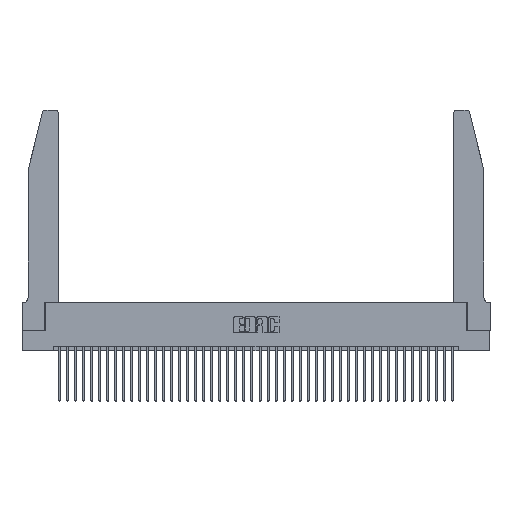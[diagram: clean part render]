
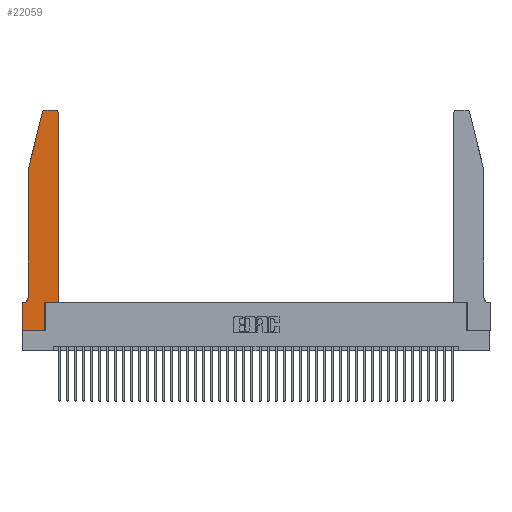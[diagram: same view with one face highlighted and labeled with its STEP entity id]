
A CAD part, top view. The second image highlights one B-rep face of the part: STEP entity #22059.
In plain terms, the highlighted planar face has unit normal (0, 0, 1).
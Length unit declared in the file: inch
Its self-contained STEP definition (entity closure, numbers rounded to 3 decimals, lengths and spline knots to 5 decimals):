
#1472 = CARTESIAN_POINT ( 'NONE',  ( 0.4505, 0.35, 0.37 ) ) ;
#2351 = ORIENTED_EDGE ( 'NONE', *, *, #39076, .T. ) ;
#2906 = DIRECTION ( 'NONE',  ( 0., -1., 0. ) ) ;
#3078 = LINE ( 'NONE', #39108, #34207 ) ;
#3206 = DIRECTION ( 'NONE',  ( 0., 0., 1. ) ) ;
#3647 = CARTESIAN_POINT ( 'NONE',  ( 0.4505, 2.72, 0.37 ) ) ;
#4287 = EDGE_CURVE ( 'NONE', #18039, #28074, #35984, .T. ) ;
#4755 = VERTEX_POINT ( 'NONE', #15818 ) ;
#5447 = LINE ( 'NONE', #38028, #14300 ) ;
#5801 = DIRECTION ( 'NONE',  ( 1., 0., 0. ) ) ;
#5887 = CARTESIAN_POINT ( 'NONE',  ( 0., 0., 0.37 ) ) ;
#7144 = CARTESIAN_POINT ( 'NONE',  ( 0.0055, 0.42, 0.37 ) ) ;
#7208 = EDGE_CURVE ( 'NONE', #29296, #27183, #28351, .T. ) ;
#7875 = DIRECTION ( 'NONE',  ( 0., 0., -1. ) ) ;
#8440 = VERTEX_POINT ( 'NONE', #33783 ) ;
#8445 = VECTOR ( 'NONE', #2906, 39.37008 ) ;
#8451 = ORIENTED_EDGE ( 'NONE', *, *, #24967, .T. ) ;
#8682 = DIRECTION ( 'NONE',  ( -1., 0., 0. ) ) ;
#8782 = CIRCLE ( 'NONE', #34345, 0.03 ) ;
#8792 = ORIENTED_EDGE ( 'NONE', *, *, #20204, .T. ) ;
#8974 = CARTESIAN_POINT ( 'NONE',  ( 0.2605, 2.75, 0.37 ) ) ;
#9156 = PLANE ( 'NONE',  #19993 ) ;
#9279 = DIRECTION ( 'NONE',  ( 0., 1., 0. ) ) ;
#9393 = VECTOR ( 'NONE', #8682, 39.37008 ) ;
#9702 = DIRECTION ( 'NONE',  ( 1., 0., 0. ) ) ;
#9722 = CARTESIAN_POINT ( 'NONE',  ( 0.4505, 0.35, 0.37 ) ) ;
#10453 = CARTESIAN_POINT ( 'NONE',  ( 0.2865, 0., 0.37 ) ) ;
#10726 = VERTEX_POINT ( 'NONE', #31061 ) ;
#10952 = VERTEX_POINT ( 'NONE', #1472 ) ;
#12100 = EDGE_LOOP ( 'NONE', ( #17981, #35621, #13462, #32931, #8792, #8451, #27539, #33921, #13154, #21253, #2351, #29216 ) ) ;
#12704 = EDGE_CURVE ( 'NONE', #29987, #22863, #8782, .T. ) ;
#13154 = ORIENTED_EDGE ( 'NONE', *, *, #7208, .T. ) ;
#13342 = VECTOR ( 'NONE', #42743, 39.37008 ) ;
#13364 = EDGE_CURVE ( 'NONE', #27407, #18039, #17043, .T. ) ;
#13462 = ORIENTED_EDGE ( 'NONE', *, *, #13364, .T. ) ;
#14059 = DIRECTION ( 'NONE',  ( -1., 0., 0. ) ) ;
#14300 = VECTOR ( 'NONE', #21576, 39.37008 ) ;
#14348 = CARTESIAN_POINT ( 'NONE',  ( 0., 0.35, 0.37 ) ) ;
#14452 = VECTOR ( 'NONE', #19868, 39.37008 ) ;
#14802 = EDGE_CURVE ( 'NONE', #19321, #10726, #39784, .T. ) ;
#15228 = EDGE_CURVE ( 'NONE', #22863, #8440, #37889, .T. ) ;
#15280 = CARTESIAN_POINT ( 'NONE',  ( 0.4205, 2.72, 0.37 ) ) ;
#15305 = VECTOR ( 'NONE', #40096, 39.37008 ) ;
#15593 = LINE ( 'NONE', #9722, #17670 ) ;
#15818 = CARTESIAN_POINT ( 'NONE',  ( 0.0055, 0.35, 0.37 ) ) ;
#16521 = EDGE_CURVE ( 'NONE', #27183, #10952, #3078, .T. ) ;
#17043 = LINE ( 'NONE', #29581, #14452 ) ;
#17247 = CARTESIAN_POINT ( 'NONE',  ( 0.0755, 0.35, 0.37 ) ) ;
#17670 = VECTOR ( 'NONE', #9279, 39.37008 ) ;
#17981 = ORIENTED_EDGE ( 'NONE', *, *, #15228, .T. ) ;
#18039 = VERTEX_POINT ( 'NONE', #24768 ) ;
#18991 = VECTOR ( 'NONE', #14059, 39.37008 ) ;
#19063 = AXIS2_PLACEMENT_3D ( 'NONE', #7144, #7875, #31136 ) ;
#19321 = VERTEX_POINT ( 'NONE', #14348 ) ;
#19694 = DIRECTION ( 'NONE',  ( 0., 0., 1. ) ) ;
#19805 = CARTESIAN_POINT ( 'NONE',  ( 0., 0.35, 0.37 ) ) ;
#19868 = DIRECTION ( 'NONE',  ( -0.239, -0.971, 0. ) ) ;
#19993 = AXIS2_PLACEMENT_3D ( 'NONE', #19805, #3206, #5801 ) ;
#20038 = CARTESIAN_POINT ( 'NONE',  ( 0.284, 2.72, 0.37 ) ) ;
#20204 = EDGE_CURVE ( 'NONE', #28074, #4755, #42888, .T. ) ;
#21104 = LINE ( 'NONE', #17247, #18991 ) ;
#21253 = ORIENTED_EDGE ( 'NONE', *, *, #16521, .T. ) ;
#21576 = DIRECTION ( 'NONE',  ( 1., 0., 0. ) ) ;
#22059 = ADVANCED_FACE ( 'NONE', ( #37833 ), #9156, .T. ) ;
#22174 = CIRCLE ( 'NONE', #38013, 0.03 ) ;
#22736 = DIRECTION ( 'NONE',  ( 1., 0., 0. ) ) ;
#22843 = CARTESIAN_POINT ( 'NONE',  ( 0.0755, 0.42, 0.37 ) ) ;
#22863 = VERTEX_POINT ( 'NONE', #23875 ) ;
#23875 = CARTESIAN_POINT ( 'NONE',  ( 0.4205, 2.75, 0.37 ) ) ;
#23933 = CARTESIAN_POINT ( 'NONE',  ( 0.0755, 2., 0.37 ) ) ;
#24768 = CARTESIAN_POINT ( 'NONE',  ( 0.0755, 2., 0.37 ) ) ;
#24967 = EDGE_CURVE ( 'NONE', #4755, #19321, #21104, .T. ) ;
#27183 = VERTEX_POINT ( 'NONE', #36464 ) ;
#27407 = VERTEX_POINT ( 'NONE', #31963 ) ;
#27539 = ORIENTED_EDGE ( 'NONE', *, *, #14802, .T. ) ;
#28074 = VERTEX_POINT ( 'NONE', #22843 ) ;
#28351 = LINE ( 'NONE', #30420, #15305 ) ;
#29216 = ORIENTED_EDGE ( 'NONE', *, *, #12704, .T. ) ;
#29296 = VERTEX_POINT ( 'NONE', #10453 ) ;
#29581 = CARTESIAN_POINT ( 'NONE',  ( 0.0755, 2., 0.37 ) ) ;
#29895 = DIRECTION ( 'NONE',  ( 0., 0., 1. ) ) ;
#29987 = VERTEX_POINT ( 'NONE', #3647 ) ;
#30420 = CARTESIAN_POINT ( 'NONE',  ( 0.2865, 0.35, 0.37 ) ) ;
#31061 = CARTESIAN_POINT ( 'NONE',  ( 0., 0., 0.37 ) ) ;
#31136 = DIRECTION ( 'NONE',  ( -1., 0., 0. ) ) ;
#31963 = CARTESIAN_POINT ( 'NONE',  ( 0.25487, 2.72718, 0.37 ) ) ;
#32931 = ORIENTED_EDGE ( 'NONE', *, *, #4287, .T. ) ;
#33783 = CARTESIAN_POINT ( 'NONE',  ( 0.284, 2.75, 0.37 ) ) ;
#33921 = ORIENTED_EDGE ( 'NONE', *, *, #42548, .T. ) ;
#34207 = VECTOR ( 'NONE', #9702, 39.37008 ) ;
#34345 = AXIS2_PLACEMENT_3D ( 'NONE', #15280, #19694, #22736 ) ;
#35621 = ORIENTED_EDGE ( 'NONE', *, *, #35917, .T. ) ;
#35917 = EDGE_CURVE ( 'NONE', #8440, #27407, #22174, .T. ) ;
#35984 = LINE ( 'NONE', #23933, #8445 ) ;
#36464 = CARTESIAN_POINT ( 'NONE',  ( 0.2865, 0.35, 0.37 ) ) ;
#37833 = FACE_OUTER_BOUND ( 'NONE', #12100, .T. ) ;
#37889 = LINE ( 'NONE', #8974, #9393 ) ;
#38013 = AXIS2_PLACEMENT_3D ( 'NONE', #20038, #29895, #39574 ) ;
#38028 = CARTESIAN_POINT ( 'NONE',  ( 0., 0., 0.37 ) ) ;
#39076 = EDGE_CURVE ( 'NONE', #10952, #29987, #15593, .T. ) ;
#39108 = CARTESIAN_POINT ( 'NONE',  ( 0.4505, 0.35, 0.37 ) ) ;
#39574 = DIRECTION ( 'NONE',  ( 1., 0., 0. ) ) ;
#39784 = LINE ( 'NONE', #5887, #13342 ) ;
#40096 = DIRECTION ( 'NONE',  ( 0., 1., 0. ) ) ;
#42548 = EDGE_CURVE ( 'NONE', #10726, #29296, #5447, .T. ) ;
#42743 = DIRECTION ( 'NONE',  ( 0., -1., 0. ) ) ;
#42888 = CIRCLE ( 'NONE', #19063, 0.07 ) ;
